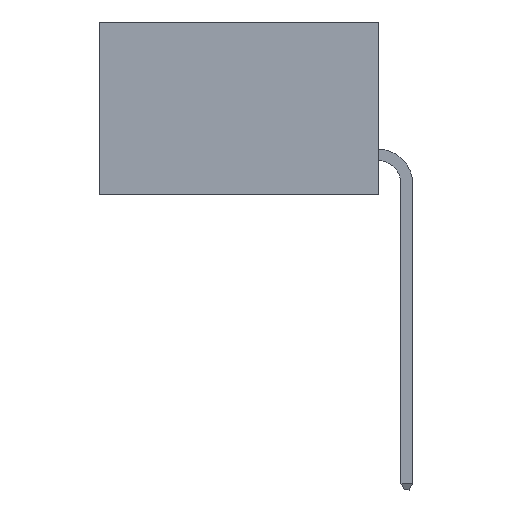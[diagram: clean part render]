
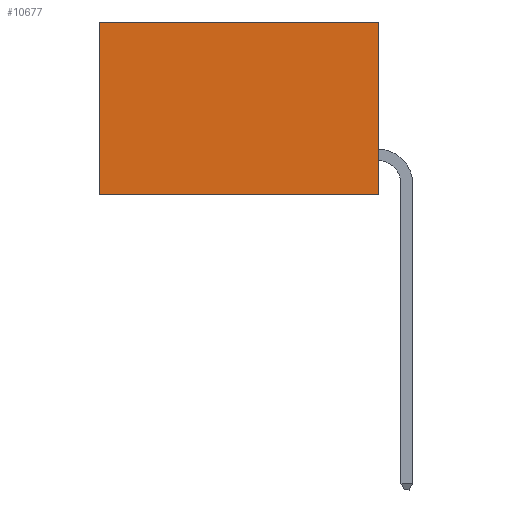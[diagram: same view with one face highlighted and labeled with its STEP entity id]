
A CAD part, left-side view. The second image highlights one B-rep face of the part: STEP entity #10677.
In plain terms, the highlighted planar face has unit normal (-1, 0, 0).
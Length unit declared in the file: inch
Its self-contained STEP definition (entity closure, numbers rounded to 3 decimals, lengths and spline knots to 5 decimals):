
#477 = PLANE ( 'NONE',  #18339 ) ;
#1071 = VECTOR ( 'NONE', #25125, 39.37008 ) ;
#2692 = DIRECTION ( 'NONE',  ( 0., 0., -1. ) ) ;
#2838 = CARTESIAN_POINT ( 'NONE',  ( 0.298, 0., 0. ) ) ;
#2953 = ORIENTED_EDGE ( 'NONE', *, *, #4512, .F. ) ;
#4512 = EDGE_CURVE ( 'NONE', #28556, #9065, #16774, .T. ) ;
#4852 = EDGE_LOOP ( 'NONE', ( #28184, #7262, #2953, #19197 ) ) ;
#6755 = LINE ( 'NONE', #21225, #13613 ) ;
#7096 = CARTESIAN_POINT ( 'NONE',  ( 0.298, 0., -0.37 ) ) ;
#7191 = CARTESIAN_POINT ( 'NONE',  ( 0.298, 0., 0. ) ) ;
#7262 = ORIENTED_EDGE ( 'NONE', *, *, #8248, .F. ) ;
#8248 = EDGE_CURVE ( 'NONE', #9065, #26120, #17295, .T. ) ;
#9065 = VERTEX_POINT ( 'NONE', #28109 ) ;
#9785 = EDGE_CURVE ( 'NONE', #28556, #18494, #15925, .T. ) ;
#10677 = ADVANCED_FACE ( 'NONE', ( #20368 ), #477, .F. ) ;
#13002 = CARTESIAN_POINT ( 'NONE',  ( 0.298, 0.6, 0. ) ) ;
#13243 = CARTESIAN_POINT ( 'NONE',  ( 0.298, 0., 0. ) ) ;
#13613 = VECTOR ( 'NONE', #18810, 39.37008 ) ;
#14201 = EDGE_CURVE ( 'NONE', #18494, #26120, #6755, .T. ) ;
#15925 = LINE ( 'NONE', #22939, #1071 ) ;
#16774 = LINE ( 'NONE', #2838, #18846 ) ;
#17295 = LINE ( 'NONE', #7096, #17998 ) ;
#17427 = CARTESIAN_POINT ( 'NONE',  ( 0.298, 0.6, -0.37 ) ) ;
#17998 = VECTOR ( 'NONE', #20353, 39.37008 ) ;
#18339 = AXIS2_PLACEMENT_3D ( 'NONE', #7191, #22490, #2692 ) ;
#18481 = DIRECTION ( 'NONE',  ( 0., 0., -1. ) ) ;
#18494 = VERTEX_POINT ( 'NONE', #13002 ) ;
#18810 = DIRECTION ( 'NONE',  ( 0., 0., -1. ) ) ;
#18846 = VECTOR ( 'NONE', #18481, 39.37008 ) ;
#19197 = ORIENTED_EDGE ( 'NONE', *, *, #9785, .T. ) ;
#20353 = DIRECTION ( 'NONE',  ( 0., 1., 0. ) ) ;
#20368 = FACE_OUTER_BOUND ( 'NONE', #4852, .T. ) ;
#21225 = CARTESIAN_POINT ( 'NONE',  ( 0.298, 0.6, 0. ) ) ;
#22490 = DIRECTION ( 'NONE',  ( 1., 0., 0. ) ) ;
#22939 = CARTESIAN_POINT ( 'NONE',  ( 0.298, 0., 0. ) ) ;
#25125 = DIRECTION ( 'NONE',  ( 0., 1., 0. ) ) ;
#26120 = VERTEX_POINT ( 'NONE', #17427 ) ;
#28109 = CARTESIAN_POINT ( 'NONE',  ( 0.298, 0., -0.37 ) ) ;
#28184 = ORIENTED_EDGE ( 'NONE', *, *, #14201, .T. ) ;
#28556 = VERTEX_POINT ( 'NONE', #13243 ) ;
